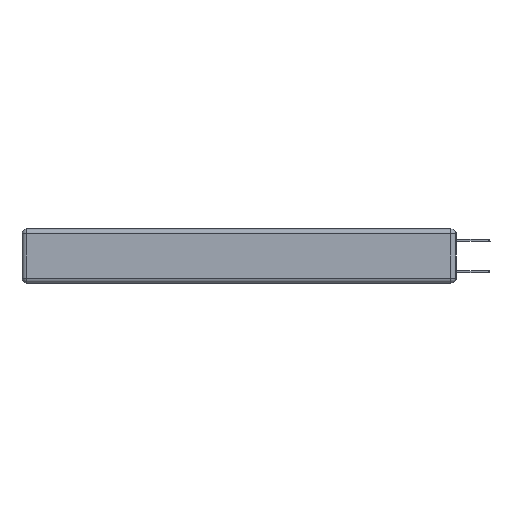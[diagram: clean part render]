
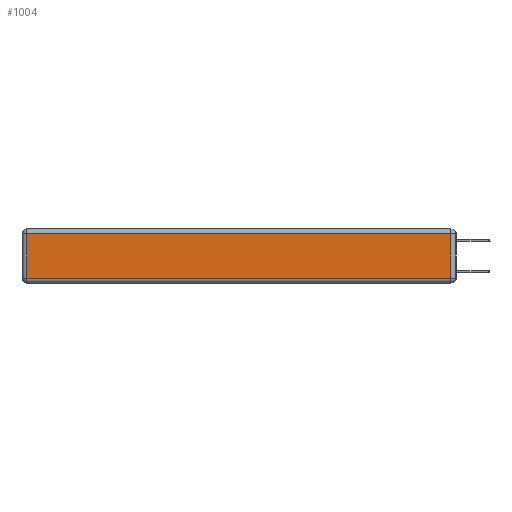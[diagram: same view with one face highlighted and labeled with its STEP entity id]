
A CAD part, left-side view. The second image highlights one B-rep face of the part: STEP entity #1004.
In plain terms, the highlighted planar face has unit normal (-1, 0, 0).
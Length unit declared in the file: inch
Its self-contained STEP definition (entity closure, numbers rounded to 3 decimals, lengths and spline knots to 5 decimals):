
#174 = AXIS2_PLACEMENT_3D ( 'NONE', #5023, #5982, #2234 ) ;
#484 = LINE ( 'NONE', #10986, #9868 ) ;
#813 = CARTESIAN_POINT ( 'NONE',  ( 0., 2.72, -0.313 ) ) ;
#1004 = ADVANCED_FACE ( 'NONE', ( #5816 ), #7986, .T. ) ;
#1380 = LINE ( 'NONE', #8628, #4560 ) ;
#1901 = LINE ( 'NONE', #8154, #11858 ) ;
#2049 = CARTESIAN_POINT ( 'NONE',  ( 0., 2.75, -0.03 ) ) ;
#2231 = DIRECTION ( 'NONE',  ( 0., 0., -1. ) ) ;
#2234 = DIRECTION ( 'NONE',  ( 0., 0., 1. ) ) ;
#3106 = DIRECTION ( 'NONE',  ( 0., -1., 0. ) ) ;
#3261 = CARTESIAN_POINT ( 'NONE',  ( 0., 0.03, -0.313 ) ) ;
#3531 = CARTESIAN_POINT ( 'NONE',  ( 0., 2.72, -0.03 ) ) ;
#3627 = EDGE_CURVE ( 'NONE', #8810, #7390, #3643, .T. ) ;
#3643 = LINE ( 'NONE', #2049, #11052 ) ;
#3718 = DIRECTION ( 'NONE',  ( 0., 0., 1. ) ) ;
#3955 = EDGE_CURVE ( 'NONE', #5121, #8810, #1380, .T. ) ;
#4102 = ORIENTED_EDGE ( 'NONE', *, *, #3955, .T. ) ;
#4560 = VECTOR ( 'NONE', #3718, 39.37008 ) ;
#4994 = ORIENTED_EDGE ( 'NONE', *, *, #8512, .T. ) ;
#5023 = CARTESIAN_POINT ( 'NONE',  ( 0., 0., -0.343 ) ) ;
#5121 = VERTEX_POINT ( 'NONE', #3261 ) ;
#5598 = EDGE_LOOP ( 'NONE', ( #4994, #4102, #11615, #7605 ) ) ;
#5816 = FACE_OUTER_BOUND ( 'NONE', #5598, .T. ) ;
#5956 = CARTESIAN_POINT ( 'NONE',  ( 0., 0.03, -0.03 ) ) ;
#5982 = DIRECTION ( 'NONE',  ( -1., 0., 0. ) ) ;
#7390 = VERTEX_POINT ( 'NONE', #3531 ) ;
#7605 = ORIENTED_EDGE ( 'NONE', *, *, #7866, .T. ) ;
#7866 = EDGE_CURVE ( 'NONE', #7390, #11604, #1901, .T. ) ;
#7986 = PLANE ( 'NONE',  #174 ) ;
#8154 = CARTESIAN_POINT ( 'NONE',  ( 0., 2.72, -0.343 ) ) ;
#8512 = EDGE_CURVE ( 'NONE', #11604, #5121, #484, .T. ) ;
#8628 = CARTESIAN_POINT ( 'NONE',  ( 0., 0.03, -0.343 ) ) ;
#8810 = VERTEX_POINT ( 'NONE', #5956 ) ;
#9096 = DIRECTION ( 'NONE',  ( 0., 1., 0. ) ) ;
#9868 = VECTOR ( 'NONE', #3106, 39.37008 ) ;
#10986 = CARTESIAN_POINT ( 'NONE',  ( 0., 0., -0.313 ) ) ;
#11052 = VECTOR ( 'NONE', #9096, 39.37008 ) ;
#11604 = VERTEX_POINT ( 'NONE', #813 ) ;
#11615 = ORIENTED_EDGE ( 'NONE', *, *, #3627, .T. ) ;
#11858 = VECTOR ( 'NONE', #2231, 39.37008 ) ;
